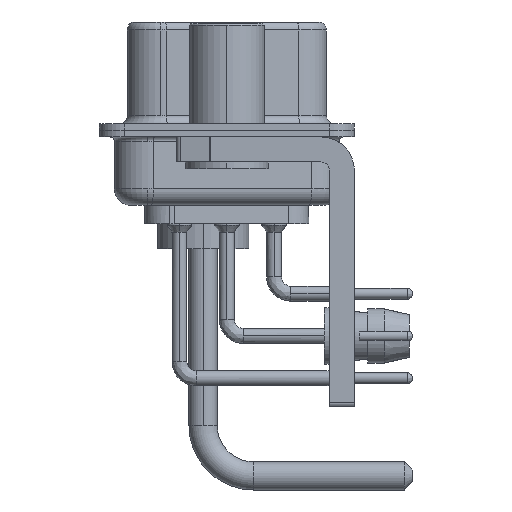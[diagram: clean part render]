
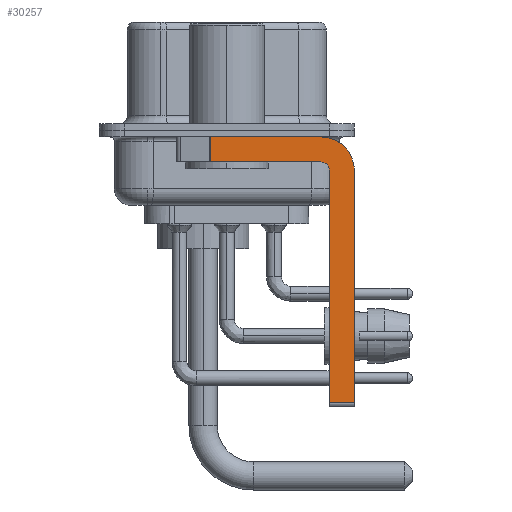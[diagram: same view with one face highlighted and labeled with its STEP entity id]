
A CAD part, left-side view. The second image highlights one B-rep face of the part: STEP entity #30257.
In plain terms, the highlighted planar face has unit normal (-1, 0, 0).
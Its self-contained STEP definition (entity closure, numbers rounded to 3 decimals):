
#128 = CARTESIAN_POINT ( 'NONE',  ( -2.9, -7.65, -2.4 ) ) ;
#573 = CARTESIAN_POINT ( 'NONE',  ( -2.9, -7.65, -2.4 ) ) ;
#591 = LINE ( 'NONE', #1422, #11835 ) ;
#752 = VECTOR ( 'NONE', #8450, 1000. ) ;
#1422 = CARTESIAN_POINT ( 'NONE',  ( -2.9, -5.65, -16.35 ) ) ;
#1817 = DIRECTION ( 'NONE',  ( 0., 0., -1. ) ) ;
#2204 = DIRECTION ( 'NONE',  ( 0., 1., 0. ) ) ;
#3880 = CIRCLE ( 'NONE', #16086, 0.5 ) ;
#4576 = VECTOR ( 'NONE', #38909, 1000. ) ;
#4797 = ORIENTED_EDGE ( 'NONE', *, *, #30019, .F. ) ;
#4832 = CARTESIAN_POINT ( 'NONE',  ( -2.9, -5.65, -2.4 ) ) ;
#6595 = EDGE_CURVE ( 'NONE', #19844, #19258, #20825, .T. ) ;
#8096 = ORIENTED_EDGE ( 'NONE', *, *, #34358, .T. ) ;
#8450 = DIRECTION ( 'NONE',  ( 0., -1., 0. ) ) ;
#11835 = VECTOR ( 'NONE', #34382, 1000. ) ;
#12033 = DIRECTION ( 'NONE',  ( 0., 0., -1. ) ) ;
#12803 = ORIENTED_EDGE ( 'NONE', *, *, #27644, .T. ) ;
#13107 = CARTESIAN_POINT ( 'NONE',  ( -2.9, 0.978, -1.9 ) ) ;
#13336 = VERTEX_POINT ( 'NONE', #573 ) ;
#13960 = CARTESIAN_POINT ( 'NONE',  ( -2.9, -5.65, -0.4 ) ) ;
#15995 = CARTESIAN_POINT ( 'NONE',  ( -2.9, -6.15, -2.4 ) ) ;
#16086 = AXIS2_PLACEMENT_3D ( 'NONE', #18135, #33781, #37211 ) ;
#16187 = CARTESIAN_POINT ( 'NONE',  ( -2.9, -5.65, -1.9 ) ) ;
#17107 = DIRECTION ( 'NONE',  ( 1., 0., 0. ) ) ;
#17681 = VECTOR ( 'NONE', #2204, 1000. ) ;
#18135 = CARTESIAN_POINT ( 'NONE',  ( -2.9, -5.65, -2.4 ) ) ;
#18443 = VERTEX_POINT ( 'NONE', #31064 ) ;
#18510 = CARTESIAN_POINT ( 'NONE',  ( -2.9, 0.978, -1.9 ) ) ;
#18980 = ORIENTED_EDGE ( 'NONE', *, *, #39774, .F. ) ;
#19258 = VERTEX_POINT ( 'NONE', #15995 ) ;
#19844 = VERTEX_POINT ( 'NONE', #26021 ) ;
#20335 = CARTESIAN_POINT ( 'NONE',  ( -2.9, -5.65, -1.9 ) ) ;
#20825 = LINE ( 'NONE', #33646, #4576 ) ;
#20908 = DIRECTION ( 'NONE',  ( 1., 0., 0. ) ) ;
#21119 = VERTEX_POINT ( 'NONE', #18510 ) ;
#21253 = AXIS2_PLACEMENT_3D ( 'NONE', #4832, #17107, #1817 ) ;
#21677 = ORIENTED_EDGE ( 'NONE', *, *, #23985, .F. ) ;
#23985 = EDGE_CURVE ( 'NONE', #37284, #13336, #30942, .T. ) ;
#24531 = AXIS2_PLACEMENT_3D ( 'NONE', #26949, #20908, #12033 ) ;
#24659 = VECTOR ( 'NONE', #37841, 1000. ) ;
#25024 = ORIENTED_EDGE ( 'NONE', *, *, #6595, .F. ) ;
#25200 = LINE ( 'NONE', #13107, #24659 ) ;
#26021 = CARTESIAN_POINT ( 'NONE',  ( -2.9, -6.15, -16.35 ) ) ;
#26179 = FACE_OUTER_BOUND ( 'NONE', #35900, .T. ) ;
#26949 = CARTESIAN_POINT ( 'NONE',  ( -2.9, -5.65, -2.4 ) ) ;
#27644 = EDGE_CURVE ( 'NONE', #18443, #21119, #25200, .T. ) ;
#27738 = LINE ( 'NONE', #128, #33295 ) ;
#28997 = EDGE_CURVE ( 'NONE', #37120, #21119, #38216, .T. ) ;
#30019 = EDGE_CURVE ( 'NONE', #19258, #37120, #3880, .T. ) ;
#30257 = ADVANCED_FACE ( 'NONE', ( #26179 ), #32382, .F. ) ;
#30942 = CIRCLE ( 'NONE', #24531, 2. ) ;
#31064 = CARTESIAN_POINT ( 'NONE',  ( -2.9, 0.978, -0.4 ) ) ;
#31708 = EDGE_CURVE ( 'NONE', #18443, #37284, #38817, .T. ) ;
#32382 = PLANE ( 'NONE',  #21253 ) ;
#32580 = ORIENTED_EDGE ( 'NONE', *, *, #31708, .F. ) ;
#32608 = CARTESIAN_POINT ( 'NONE',  ( -2.9, -7.65, -16.35 ) ) ;
#33295 = VECTOR ( 'NONE', #36951, 1000. ) ;
#33646 = CARTESIAN_POINT ( 'NONE',  ( -2.9, -6.15, -16.6 ) ) ;
#33781 = DIRECTION ( 'NONE',  ( -1., 0., 0. ) ) ;
#34358 = EDGE_CURVE ( 'NONE', #19844, #39142, #591, .T. ) ;
#34382 = DIRECTION ( 'NONE',  ( 0., -1., 0. ) ) ;
#35711 = ORIENTED_EDGE ( 'NONE', *, *, #28997, .F. ) ;
#35900 = EDGE_LOOP ( 'NONE', ( #32580, #12803, #35711, #4797, #25024, #8096, #18980, #21677 ) ) ;
#36951 = DIRECTION ( 'NONE',  ( 0., 0., -1. ) ) ;
#37120 = VERTEX_POINT ( 'NONE', #16187 ) ;
#37211 = DIRECTION ( 'NONE',  ( 0., 0., 1. ) ) ;
#37284 = VERTEX_POINT ( 'NONE', #13960 ) ;
#37841 = DIRECTION ( 'NONE',  ( 0., 0., -1. ) ) ;
#38216 = LINE ( 'NONE', #20335, #17681 ) ;
#38618 = CARTESIAN_POINT ( 'NONE',  ( -2.9, 3., -0.4 ) ) ;
#38817 = LINE ( 'NONE', #38618, #752 ) ;
#38909 = DIRECTION ( 'NONE',  ( 0., 0., 1. ) ) ;
#39142 = VERTEX_POINT ( 'NONE', #32608 ) ;
#39774 = EDGE_CURVE ( 'NONE', #13336, #39142, #27738, .T. ) ;
